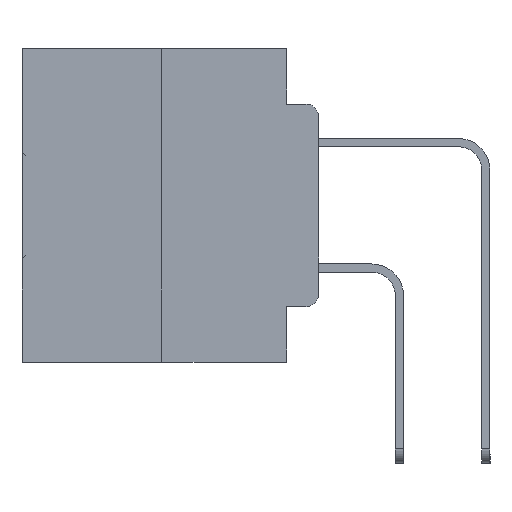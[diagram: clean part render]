
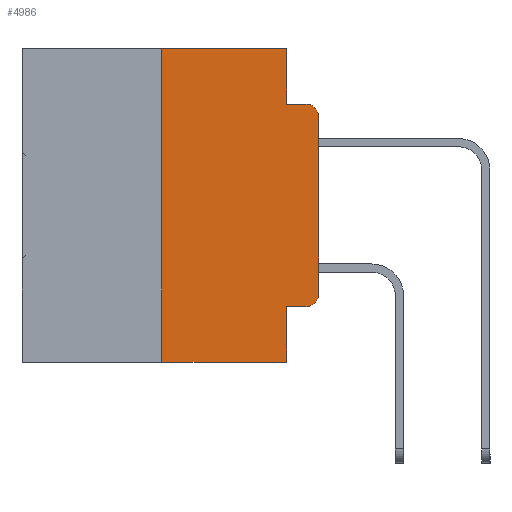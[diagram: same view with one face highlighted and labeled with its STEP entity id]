
A CAD part, left-side view. The second image highlights one B-rep face of the part: STEP entity #4986.
In plain terms, the highlighted planar face has unit normal (-1, 0, 0).
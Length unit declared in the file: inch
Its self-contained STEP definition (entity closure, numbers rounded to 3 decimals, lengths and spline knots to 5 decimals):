
#137 = ORIENTED_EDGE ( 'NONE', *, *, #8187, .F. ) ;
#601 = ORIENTED_EDGE ( 'NONE', *, *, #12709, .T. ) ;
#640 = CARTESIAN_POINT ( 'NONE',  ( 0., 0.473, 0. ) ) ;
#1382 = CARTESIAN_POINT ( 'NONE',  ( 0., 0.051, -0.0885 ) ) ;
#1384 = AXIS2_PLACEMENT_3D ( 'NONE', #7086, #25087, #9663 ) ;
#1593 = EDGE_CURVE ( 'NONE', #11371, #25235, #8074, .T. ) ;
#2073 = CARTESIAN_POINT ( 'NONE',  ( 0., 0.051, 0. ) ) ;
#2108 = VERTEX_POINT ( 'NONE', #17888 ) ;
#2222 = CARTESIAN_POINT ( 'NONE',  ( 0., 0.473, 0. ) ) ;
#2911 = DIRECTION ( 'NONE',  ( -1., 0., 0. ) ) ;
#2921 = CARTESIAN_POINT ( 'NONE',  ( 0., 0., -0.3915 ) ) ;
#3480 = LINE ( 'NONE', #24144, #16452 ) ;
#3603 = DIRECTION ( 'NONE',  ( 0., 0., -1. ) ) ;
#4733 = CARTESIAN_POINT ( 'NONE',  ( 0., 0.051, 0. ) ) ;
#4986 = ADVANCED_FACE ( 'NONE', ( #26076 ), #5945, .F. ) ;
#5213 = DIRECTION ( 'NONE',  ( 0., 0., 1. ) ) ;
#5521 = VERTEX_POINT ( 'NONE', #2921 ) ;
#5945 = PLANE ( 'NONE',  #31347 ) ;
#6445 = EDGE_CURVE ( 'NONE', #13005, #11419, #20320, .T. ) ;
#7086 = CARTESIAN_POINT ( 'NONE',  ( 0., 0.02, -0.1085 ) ) ;
#7406 = DIRECTION ( 'NONE',  ( 0., -1., 0. ) ) ;
#7511 = ORIENTED_EDGE ( 'NONE', *, *, #29093, .T. ) ;
#8074 = LINE ( 'NONE', #25078, #14099 ) ;
#8155 = VERTEX_POINT ( 'NONE', #2073 ) ;
#8187 = EDGE_CURVE ( 'NONE', #11371, #11829, #12252, .T. ) ;
#8562 = DIRECTION ( 'NONE',  ( 0., 0., -1. ) ) ;
#8931 = LINE ( 'NONE', #29959, #14950 ) ;
#9132 = ORIENTED_EDGE ( 'NONE', *, *, #6445, .F. ) ;
#9322 = VECTOR ( 'NONE', #5213, 39.37008 ) ;
#9663 = DIRECTION ( 'NONE',  ( 0., 0., -1. ) ) ;
#10093 = EDGE_CURVE ( 'NONE', #5521, #23342, #8931, .T. ) ;
#10967 = EDGE_CURVE ( 'NONE', #2108, #32710, #21376, .T. ) ;
#11371 = VERTEX_POINT ( 'NONE', #17168 ) ;
#11419 = VERTEX_POINT ( 'NONE', #30201 ) ;
#11829 = VERTEX_POINT ( 'NONE', #32940 ) ;
#11882 = DIRECTION ( 'NONE',  ( 0., -1., 0. ) ) ;
#11999 = EDGE_CURVE ( 'NONE', #2108, #11829, #31763, .T. ) ;
#12252 = LINE ( 'NONE', #4733, #17519 ) ;
#12709 = EDGE_CURVE ( 'NONE', #25235, #5521, #25314, .T. ) ;
#12909 = EDGE_CURVE ( 'NONE', #8155, #13005, #3480, .T. ) ;
#12940 = CARTESIAN_POINT ( 'NONE',  ( 0., 0.473, -0.5 ) ) ;
#13005 = VERTEX_POINT ( 'NONE', #1382 ) ;
#14099 = VECTOR ( 'NONE', #11882, 39.37008 ) ;
#14370 = ORIENTED_EDGE ( 'NONE', *, *, #10967, .F. ) ;
#14950 = VECTOR ( 'NONE', #24891, 39.37008 ) ;
#16452 = VECTOR ( 'NONE', #3603, 39.37008 ) ;
#16513 = VECTOR ( 'NONE', #18145, 39.37008 ) ;
#16792 = ORIENTED_EDGE ( 'NONE', *, *, #12909, .F. ) ;
#16858 = ORIENTED_EDGE ( 'NONE', *, *, #1593, .T. ) ;
#17168 = CARTESIAN_POINT ( 'NONE',  ( 0., 0.051, -0.4115 ) ) ;
#17519 = VECTOR ( 'NONE', #27961, 39.37008 ) ;
#17888 = CARTESIAN_POINT ( 'NONE',  ( 0., 0.25, -0.5 ) ) ;
#18017 = CARTESIAN_POINT ( 'NONE',  ( 0., 0., -0.1085 ) ) ;
#18043 = CIRCLE ( 'NONE', #1384, 0.02 ) ;
#18145 = DIRECTION ( 'NONE',  ( 0., -1., 0. ) ) ;
#18429 = CARTESIAN_POINT ( 'NONE',  ( 0., 0.02, -0.3915 ) ) ;
#19628 = ORIENTED_EDGE ( 'NONE', *, *, #29737, .F. ) ;
#19726 = AXIS2_PLACEMENT_3D ( 'NONE', #18429, #2911, #20997 ) ;
#20320 = LINE ( 'NONE', #28298, #33158 ) ;
#20692 = CARTESIAN_POINT ( 'NONE',  ( 0., 0.02, -0.4115 ) ) ;
#20997 = DIRECTION ( 'NONE',  ( 0., 0., -1. ) ) ;
#21376 = LINE ( 'NONE', #28446, #9322 ) ;
#21570 = VECTOR ( 'NONE', #7406, 39.37008 ) ;
#22670 = CARTESIAN_POINT ( 'NONE',  ( 0., 0.25, 0. ) ) ;
#22821 = ORIENTED_EDGE ( 'NONE', *, *, #11999, .T. ) ;
#23342 = VERTEX_POINT ( 'NONE', #18017 ) ;
#23972 = DIRECTION ( 'NONE',  ( 1., 0., 0. ) ) ;
#24144 = CARTESIAN_POINT ( 'NONE',  ( 0., 0.051, 0. ) ) ;
#24891 = DIRECTION ( 'NONE',  ( 0., 0., 1. ) ) ;
#25078 = CARTESIAN_POINT ( 'NONE',  ( 0., 0.051, -0.4115 ) ) ;
#25087 = DIRECTION ( 'NONE',  ( -1., 0., 0. ) ) ;
#25235 = VERTEX_POINT ( 'NONE', #20692 ) ;
#25314 = CIRCLE ( 'NONE', #19726, 0.02 ) ;
#25980 = EDGE_LOOP ( 'NONE', ( #28823, #7511, #9132, #16792, #19628, #14370, #22821, #137, #16858, #601 ) ) ;
#26076 = FACE_OUTER_BOUND ( 'NONE', #25980, .T. ) ;
#26836 = LINE ( 'NONE', #2222, #21570 ) ;
#27961 = DIRECTION ( 'NONE',  ( 0., 0., -1. ) ) ;
#28298 = CARTESIAN_POINT ( 'NONE',  ( 0., 0.051, -0.0885 ) ) ;
#28446 = CARTESIAN_POINT ( 'NONE',  ( 0., 0.25, 0. ) ) ;
#28823 = ORIENTED_EDGE ( 'NONE', *, *, #10093, .T. ) ;
#29093 = EDGE_CURVE ( 'NONE', #23342, #11419, #18043, .T. ) ;
#29737 = EDGE_CURVE ( 'NONE', #32710, #8155, #26836, .T. ) ;
#29959 = CARTESIAN_POINT ( 'NONE',  ( 0., 0., 0. ) ) ;
#30201 = CARTESIAN_POINT ( 'NONE',  ( 0., 0.02, -0.0885 ) ) ;
#30859 = DIRECTION ( 'NONE',  ( 0., -1., 0. ) ) ;
#31347 = AXIS2_PLACEMENT_3D ( 'NONE', #640, #23972, #8562 ) ;
#31763 = LINE ( 'NONE', #12940, #16513 ) ;
#32710 = VERTEX_POINT ( 'NONE', #22670 ) ;
#32940 = CARTESIAN_POINT ( 'NONE',  ( 0., 0.051, -0.5 ) ) ;
#33158 = VECTOR ( 'NONE', #30859, 39.37008 ) ;
